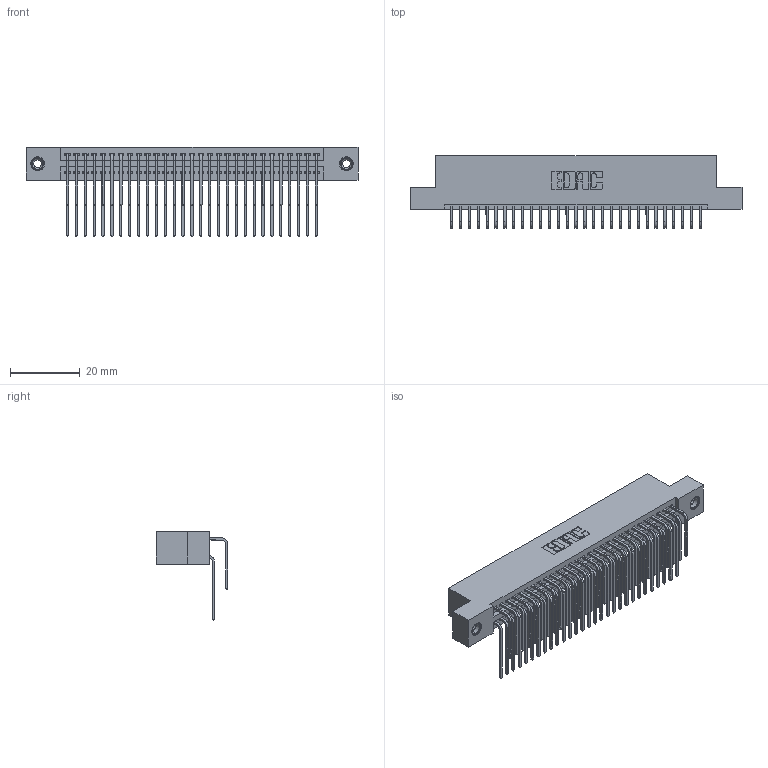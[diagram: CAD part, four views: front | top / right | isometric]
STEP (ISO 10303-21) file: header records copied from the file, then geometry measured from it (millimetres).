
FILE_DESCRIPTION (( 'STEP AP203' ), '1' );
FILE_NAME ('395-058-559-208.STEP', '2019-10-23T13:06:18', ( '' ), ( '' ), 'SwSTEP 2.0', 'SolidWorks 2016', '' );
FILE_SCHEMA (( 'CONFIG_CONTROL_DESIGN' ));
Length unit declared in the file: inch
Products named in the file (5): 345-250-001_345-250-003-102; 395-058-559-208; 345 Part_Flush Mounting Lugs - 0.156 Dia-TI; 345-292-001_558 559 Tail - 1; 345-292-001_559 Tail - 2
Assembly tree (61 placements, depth 2):
  395-058-559-208
    345 Part_Flush Mounting Lugs - 0.156 Dia-TI
    345-292-001_558 559 Tail - 1  x29
    345-292-001_559 Tail - 2  x29
    345-250-001_345-250-003-102  x2
Bounding box: 94.87 x 20.56 x 25.53 mm (x, y, z)
Volume: 9423.1 mm3; surface area: 15263.9 mm2
Topology: 61 solids, 61 shells, 3202 faces, 9467 edges, 6226 vertices
Faces by surface type: plane 2142, cylinder 1044, cone 12, torus 4
Entity records: 27342 total; most frequent: CARTESIAN_POINT 4622, ORIENTED_EDGE 4498, DIRECTION 4091, EDGE_CURVE 2249, VECTOR 1941, LINE 1941, VERTEX_POINT 1492, AXIS2_PLACEMENT_3D 1075
